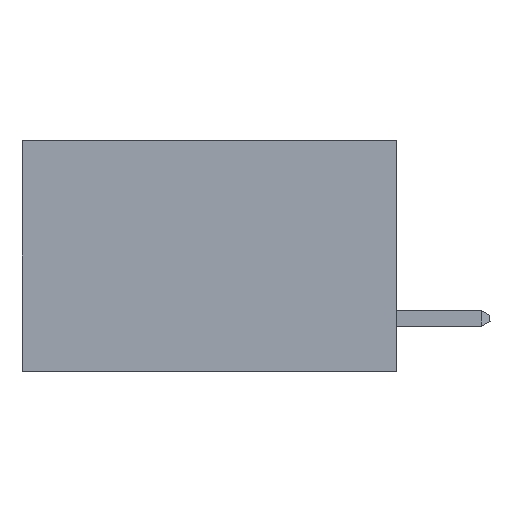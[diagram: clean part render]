
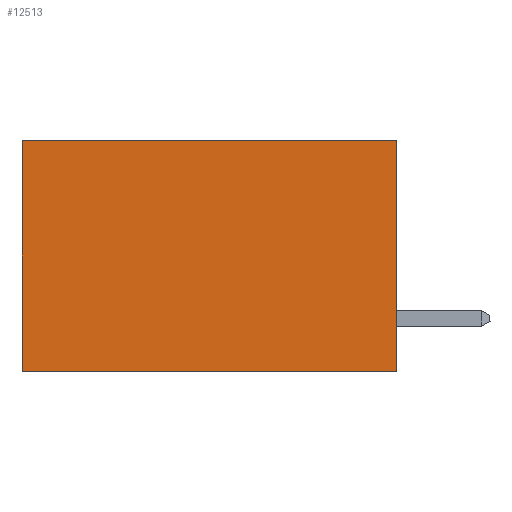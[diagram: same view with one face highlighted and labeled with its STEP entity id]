
A CAD part, left-side view. The second image highlights one B-rep face of the part: STEP entity #12513.
In plain terms, the highlighted planar face has unit normal (-1, 0, 0).
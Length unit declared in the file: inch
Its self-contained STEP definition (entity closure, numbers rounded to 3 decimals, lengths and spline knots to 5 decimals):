
#81 = VERTEX_POINT ( 'NONE', #13849 ) ;
#330 = CARTESIAN_POINT ( 'NONE',  ( 0.298, 0., 0. ) ) ;
#721 = LINE ( 'NONE', #14783, #15197 ) ;
#1718 = VECTOR ( 'NONE', #10799, 39.37008 ) ;
#2239 = CARTESIAN_POINT ( 'NONE',  ( 0.298, 0., -0.37 ) ) ;
#2747 = EDGE_CURVE ( 'NONE', #4636, #81, #2875, .T. ) ;
#2875 = LINE ( 'NONE', #15537, #6198 ) ;
#4220 = DIRECTION ( 'NONE',  ( 0., 1., 0. ) ) ;
#4348 = VERTEX_POINT ( 'NONE', #2239 ) ;
#4636 = VERTEX_POINT ( 'NONE', #330 ) ;
#4867 = EDGE_CURVE ( 'NONE', #4348, #15599, #7271, .T. ) ;
#6073 = CARTESIAN_POINT ( 'NONE',  ( 0.298, 0., 0. ) ) ;
#6198 = VECTOR ( 'NONE', #11413, 39.37008 ) ;
#7271 = LINE ( 'NONE', #13052, #10593 ) ;
#7513 = PLANE ( 'NONE',  #10862 ) ;
#7562 = ORIENTED_EDGE ( 'NONE', *, *, #2747, .T. ) ;
#7678 = EDGE_LOOP ( 'NONE', ( #9052, #11666, #12110, #7562 ) ) ;
#8947 = DIRECTION ( 'NONE',  ( 0., 0., -1. ) ) ;
#9052 = ORIENTED_EDGE ( 'NONE', *, *, #12741, .T. ) ;
#9404 = CARTESIAN_POINT ( 'NONE',  ( 0.298, 0.6, 0. ) ) ;
#9775 = LINE ( 'NONE', #9404, #1718 ) ;
#10593 = VECTOR ( 'NONE', #4220, 39.37008 ) ;
#10799 = DIRECTION ( 'NONE',  ( 0., 0., -1. ) ) ;
#10862 = AXIS2_PLACEMENT_3D ( 'NONE', #6073, #17120, #8947 ) ;
#11113 = EDGE_CURVE ( 'NONE', #4636, #4348, #721, .T. ) ;
#11413 = DIRECTION ( 'NONE',  ( 0., 1., 0. ) ) ;
#11628 = CARTESIAN_POINT ( 'NONE',  ( 0.298, 0.6, -0.37 ) ) ;
#11666 = ORIENTED_EDGE ( 'NONE', *, *, #4867, .F. ) ;
#12110 = ORIENTED_EDGE ( 'NONE', *, *, #11113, .F. ) ;
#12513 = ADVANCED_FACE ( 'NONE', ( #16362 ), #7513, .F. ) ;
#12741 = EDGE_CURVE ( 'NONE', #81, #15599, #9775, .T. ) ;
#13052 = CARTESIAN_POINT ( 'NONE',  ( 0.298, 0., -0.37 ) ) ;
#13849 = CARTESIAN_POINT ( 'NONE',  ( 0.298, 0.6, 0. ) ) ;
#14783 = CARTESIAN_POINT ( 'NONE',  ( 0.298, 0., 0. ) ) ;
#15197 = VECTOR ( 'NONE', #17486, 39.37008 ) ;
#15537 = CARTESIAN_POINT ( 'NONE',  ( 0.298, 0., 0. ) ) ;
#15599 = VERTEX_POINT ( 'NONE', #11628 ) ;
#16362 = FACE_OUTER_BOUND ( 'NONE', #7678, .T. ) ;
#17120 = DIRECTION ( 'NONE',  ( 1., 0., 0. ) ) ;
#17486 = DIRECTION ( 'NONE',  ( 0., 0., -1. ) ) ;
